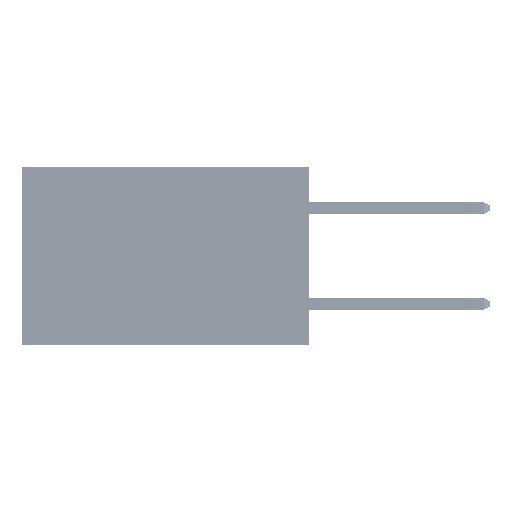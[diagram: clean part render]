
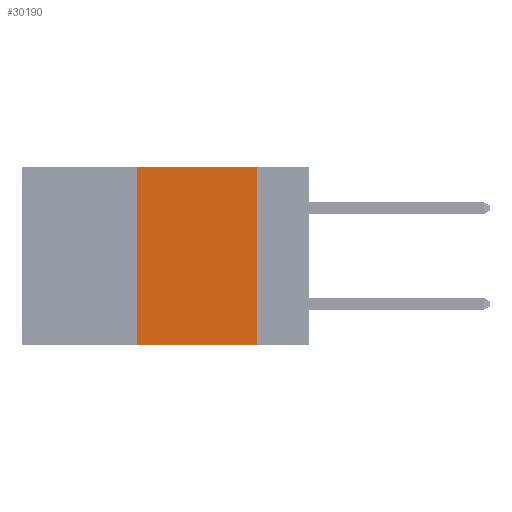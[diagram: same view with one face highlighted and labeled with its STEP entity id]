
A CAD part, left-side view. The second image highlights one B-rep face of the part: STEP entity #30190.
In plain terms, the highlighted planar face has unit normal (-1, 0, 0).
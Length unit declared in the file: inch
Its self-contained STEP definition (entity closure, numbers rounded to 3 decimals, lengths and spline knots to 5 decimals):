
#1804 = ORIENTED_EDGE ( 'NONE', *, *, #6981, .F. ) ;
#1967 = ORIENTED_EDGE ( 'NONE', *, *, #13391, .F. ) ;
#4906 = FACE_OUTER_BOUND ( 'NONE', #12421, .T. ) ;
#6981 = EDGE_CURVE ( 'NONE', #48005, #12195, #29097, .T. ) ;
#7605 = DIRECTION ( 'NONE',  ( 0., 0., -1. ) ) ;
#8274 = CARTESIAN_POINT ( 'NONE',  ( 0., 0.6, -0.37 ) ) ;
#8553 = CARTESIAN_POINT ( 'NONE',  ( 0., 0.6, 0. ) ) ;
#9189 = VECTOR ( 'NONE', #39997, 39.37008 ) ;
#10559 = AXIS2_PLACEMENT_3D ( 'NONE', #8553, #45820, #34992 ) ;
#12195 = VERTEX_POINT ( 'NONE', #24098 ) ;
#12269 = VERTEX_POINT ( 'NONE', #47092 ) ;
#12421 = EDGE_LOOP ( 'NONE', ( #1967, #15869, #1804, #34681 ) ) ;
#13391 = EDGE_CURVE ( 'NONE', #12269, #47813, #29424, .T. ) ;
#13932 = VECTOR ( 'NONE', #45877, 39.37008 ) ;
#14459 = CARTESIAN_POINT ( 'NONE',  ( 0., 0.11, -0.37 ) ) ;
#15869 = ORIENTED_EDGE ( 'NONE', *, *, #45180, .F. ) ;
#19693 = VECTOR ( 'NONE', #26436, 39.37008 ) ;
#23194 = CARTESIAN_POINT ( 'NONE',  ( 0., 0.11, 0. ) ) ;
#23651 = PLANE ( 'NONE',  #10559 ) ;
#23895 = LINE ( 'NONE', #8274, #13932 ) ;
#24098 = CARTESIAN_POINT ( 'NONE',  ( 0., 0.36, 0. ) ) ;
#26436 = DIRECTION ( 'NONE',  ( 0., 0., 1. ) ) ;
#28034 = CARTESIAN_POINT ( 'NONE',  ( 0., 0.6, 0. ) ) ;
#28225 = VECTOR ( 'NONE', #7605, 39.37008 ) ;
#29097 = LINE ( 'NONE', #41394, #19693 ) ;
#29424 = LINE ( 'NONE', #23194, #28225 ) ;
#30190 = ADVANCED_FACE ( 'NONE', ( #4906 ), #23651, .F. ) ;
#34211 = EDGE_CURVE ( 'NONE', #48005, #47813, #23895, .T. ) ;
#34681 = ORIENTED_EDGE ( 'NONE', *, *, #34211, .T. ) ;
#34992 = DIRECTION ( 'NONE',  ( 0., 0., -1. ) ) ;
#35625 = LINE ( 'NONE', #28034, #9189 ) ;
#38807 = CARTESIAN_POINT ( 'NONE',  ( 0., 0.36, -0.37 ) ) ;
#39997 = DIRECTION ( 'NONE',  ( 0., -1., 0. ) ) ;
#41394 = CARTESIAN_POINT ( 'NONE',  ( 0., 0.36, 0. ) ) ;
#45180 = EDGE_CURVE ( 'NONE', #12195, #12269, #35625, .T. ) ;
#45820 = DIRECTION ( 'NONE',  ( 1., 0., 0. ) ) ;
#45877 = DIRECTION ( 'NONE',  ( 0., -1., 0. ) ) ;
#47092 = CARTESIAN_POINT ( 'NONE',  ( 0., 0.11, 0. ) ) ;
#47813 = VERTEX_POINT ( 'NONE', #14459 ) ;
#48005 = VERTEX_POINT ( 'NONE', #38807 ) ;
